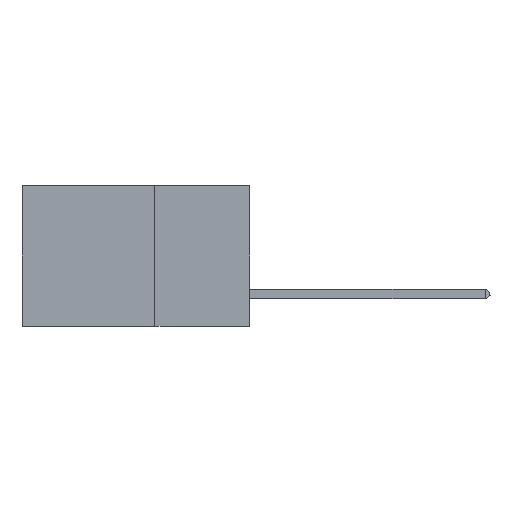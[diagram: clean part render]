
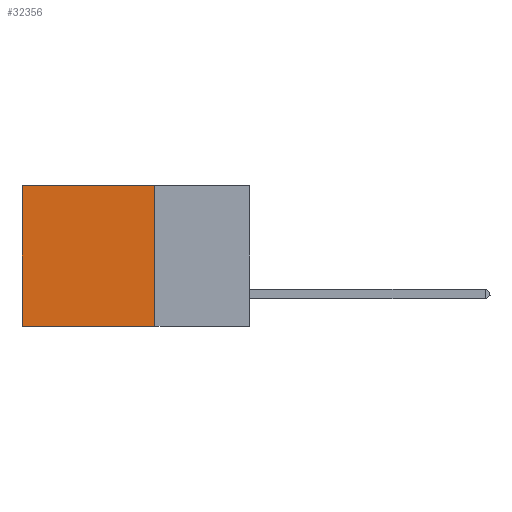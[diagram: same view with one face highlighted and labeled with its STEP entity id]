
A CAD part, left-side view. The second image highlights one B-rep face of the part: STEP entity #32356.
In plain terms, the highlighted planar face has unit normal (-1, 0, 0).
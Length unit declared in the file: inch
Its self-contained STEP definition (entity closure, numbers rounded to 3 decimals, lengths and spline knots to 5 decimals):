
#180 = VERTEX_POINT ( 'NONE', #31421 ) ;
#1788 = EDGE_CURVE ( 'NONE', #2330, #48132, #13662, .T. ) ;
#2330 = VERTEX_POINT ( 'NONE', #15619 ) ;
#5974 = PLANE ( 'NONE',  #7798 ) ;
#7306 = LINE ( 'NONE', #40047, #34051 ) ;
#7798 = AXIS2_PLACEMENT_3D ( 'NONE', #18169, #14257, #21866 ) ;
#7929 = DIRECTION ( 'NONE',  ( 0., 0., -1. ) ) ;
#8383 = ORIENTED_EDGE ( 'NONE', *, *, #1788, .F. ) ;
#9599 = CARTESIAN_POINT ( 'NONE',  ( 0.2875, 0.25, -0.37 ) ) ;
#10986 = ORIENTED_EDGE ( 'NONE', *, *, #12074, .T. ) ;
#12074 = EDGE_CURVE ( 'NONE', #2330, #44597, #7306, .T. ) ;
#13662 = LINE ( 'NONE', #29595, #22720 ) ;
#14257 = DIRECTION ( 'NONE',  ( 1., 0., 0. ) ) ;
#15232 = CARTESIAN_POINT ( 'NONE',  ( 0.2875, 0.6, 0. ) ) ;
#15619 = CARTESIAN_POINT ( 'NONE',  ( 0.2875, 0.25, 0. ) ) ;
#18132 = VECTOR ( 'NONE', #36563, 39.37008 ) ;
#18169 = CARTESIAN_POINT ( 'NONE',  ( 0.2875, 0.25, 0. ) ) ;
#20962 = LINE ( 'NONE', #15232, #41623 ) ;
#21088 = FACE_OUTER_BOUND ( 'NONE', #39609, .T. ) ;
#21866 = DIRECTION ( 'NONE',  ( 0., 0., -1. ) ) ;
#22720 = VECTOR ( 'NONE', #33045, 39.37008 ) ;
#27853 = ORIENTED_EDGE ( 'NONE', *, *, #47954, .F. ) ;
#29541 = CARTESIAN_POINT ( 'NONE',  ( 0.2875, 0.25, -0.37 ) ) ;
#29595 = CARTESIAN_POINT ( 'NONE',  ( 0.2875, 0.25, 0. ) ) ;
#30691 = ORIENTED_EDGE ( 'NONE', *, *, #49529, .T. ) ;
#31421 = CARTESIAN_POINT ( 'NONE',  ( 0.2875, 0.6, -0.37 ) ) ;
#32356 = ADVANCED_FACE ( 'NONE', ( #21088 ), #5974, .F. ) ;
#32413 = CARTESIAN_POINT ( 'NONE',  ( 0.2875, 0.6, 0. ) ) ;
#33045 = DIRECTION ( 'NONE',  ( 0., 0., -1. ) ) ;
#34051 = VECTOR ( 'NONE', #44070, 39.37008 ) ;
#36563 = DIRECTION ( 'NONE',  ( 0., 1., 0. ) ) ;
#38781 = LINE ( 'NONE', #9599, #18132 ) ;
#39609 = EDGE_LOOP ( 'NONE', ( #30691, #27853, #8383, #10986 ) ) ;
#40047 = CARTESIAN_POINT ( 'NONE',  ( 0.2875, 0.25, 0. ) ) ;
#41623 = VECTOR ( 'NONE', #7929, 39.37008 ) ;
#44070 = DIRECTION ( 'NONE',  ( 0., 1., 0. ) ) ;
#44597 = VERTEX_POINT ( 'NONE', #32413 ) ;
#47954 = EDGE_CURVE ( 'NONE', #48132, #180, #38781, .T. ) ;
#48132 = VERTEX_POINT ( 'NONE', #29541 ) ;
#49529 = EDGE_CURVE ( 'NONE', #44597, #180, #20962, .T. ) ;
